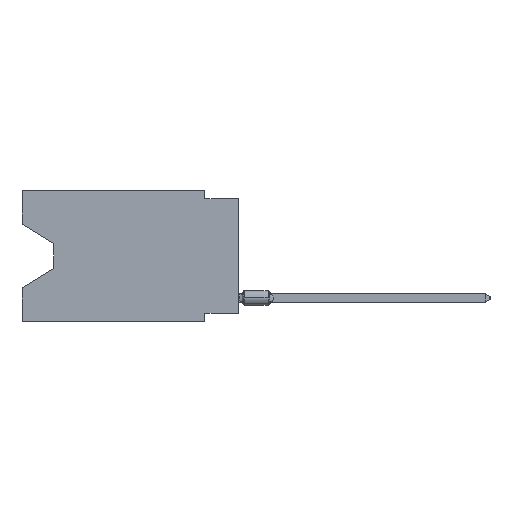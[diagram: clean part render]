
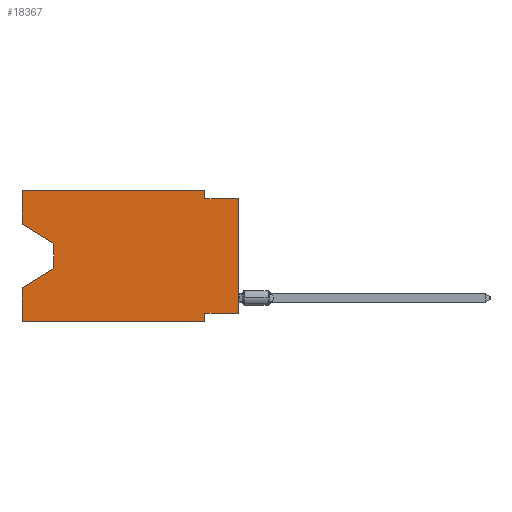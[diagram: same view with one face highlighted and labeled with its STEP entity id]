
A CAD part, left-side view. The second image highlights one B-rep face of the part: STEP entity #18367.
In plain terms, the highlighted planar face has unit normal (-1, 0, 0).
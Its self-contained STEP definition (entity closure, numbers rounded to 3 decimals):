
#168 = ORIENTED_EDGE ( 'NONE', *, *, #15667, .F. ) ;
#185 = VECTOR ( 'NONE', #19411, 1000. ) ;
#812 = VERTEX_POINT ( 'NONE', #38391 ) ;
#916 = VECTOR ( 'NONE', #42752, 1000. ) ;
#1492 = DIRECTION ( 'NONE',  ( 0., -1., 0. ) ) ;
#3178 = VERTEX_POINT ( 'NONE', #38609 ) ;
#3614 = CARTESIAN_POINT ( 'NONE',  ( 0., 0., -0.635 ) ) ;
#3881 = VERTEX_POINT ( 'NONE', #13965 ) ;
#4156 = EDGE_CURVE ( 'NONE', #30606, #30256, #38483, .T. ) ;
#4614 = CARTESIAN_POINT ( 'NONE',  ( 0., 16.383, -9.906 ) ) ;
#5006 = ORIENTED_EDGE ( 'NONE', *, *, #40846, .T. ) ;
#6402 = LINE ( 'NONE', #41507, #27598 ) ;
#7104 = VERTEX_POINT ( 'NONE', #14710 ) ;
#7480 = VECTOR ( 'NONE', #28845, 1000. ) ;
#7655 = LINE ( 'NONE', #31886, #916 ) ;
#8007 = EDGE_CURVE ( 'NONE', #7104, #30606, #35783, .T. ) ;
#8236 = CARTESIAN_POINT ( 'NONE',  ( 0., 16.383, -2.546 ) ) ;
#8937 = DIRECTION ( 'NONE',  ( 1., 0., 0. ) ) ;
#8999 = ORIENTED_EDGE ( 'NONE', *, *, #39989, .T. ) ;
#9164 = FACE_OUTER_BOUND ( 'NONE', #39672, .T. ) ;
#9329 = CARTESIAN_POINT ( 'NONE',  ( 0., 2.54, -9.271 ) ) ;
#9540 = ORIENTED_EDGE ( 'NONE', *, *, #4156, .F. ) ;
#9961 = ORIENTED_EDGE ( 'NONE', *, *, #20141, .F. ) ;
#10721 = DIRECTION ( 'NONE',  ( 0., -1., 0. ) ) ;
#10943 = LINE ( 'NONE', #42808, #21539 ) ;
#11065 = VECTOR ( 'NONE', #10721, 1000. ) ;
#12923 = VERTEX_POINT ( 'NONE', #24938 ) ;
#13878 = ORIENTED_EDGE ( 'NONE', *, *, #44050, .T. ) ;
#13965 = CARTESIAN_POINT ( 'NONE',  ( 0., 13.97, -4.013 ) ) ;
#14253 = DIRECTION ( 'NONE',  ( 0., -1., 0. ) ) ;
#14710 = CARTESIAN_POINT ( 'NONE',  ( 0., 2.54, 0. ) ) ;
#15667 = EDGE_CURVE ( 'NONE', #42163, #3178, #26783, .T. ) ;
#16546 = PLANE ( 'NONE',  #26722 ) ;
#16967 = ORIENTED_EDGE ( 'NONE', *, *, #26212, .T. ) ;
#17009 = CARTESIAN_POINT ( 'NONE',  ( 0., 16.383, 0. ) ) ;
#17024 = DIRECTION ( 'NONE',  ( 0., 0.855, -0.519 ) ) ;
#17394 = VECTOR ( 'NONE', #34828, 1000. ) ;
#17498 = LINE ( 'NONE', #27440, #17394 ) ;
#18367 = ADVANCED_FACE ( 'NONE', ( #9164 ), #16546, .F. ) ;
#19096 = ORIENTED_EDGE ( 'NONE', *, *, #8007, .F. ) ;
#19411 = DIRECTION ( 'NONE',  ( 0., 0., 1. ) ) ;
#19811 = EDGE_CURVE ( 'NONE', #23312, #12923, #17498, .T. ) ;
#20141 = EDGE_CURVE ( 'NONE', #812, #43553, #26247, .T. ) ;
#21539 = VECTOR ( 'NONE', #39777, 1000. ) ;
#21571 = LINE ( 'NONE', #42586, #11065 ) ;
#22924 = ORIENTED_EDGE ( 'NONE', *, *, #26256, .F. ) ;
#23024 = DIRECTION ( 'NONE',  ( 0., 0., 1. ) ) ;
#23312 = VERTEX_POINT ( 'NONE', #9329 ) ;
#24254 = VECTOR ( 'NONE', #14253, 1000. ) ;
#24682 = CARTESIAN_POINT ( 'NONE',  ( 0., 2.54, -0.635 ) ) ;
#24904 = CARTESIAN_POINT ( 'NONE',  ( 0., 16.383, 0. ) ) ;
#24938 = CARTESIAN_POINT ( 'NONE',  ( 0., 2.54, -9.906 ) ) ;
#26212 = EDGE_CURVE ( 'NONE', #32530, #3178, #30872, .T. ) ;
#26247 = LINE ( 'NONE', #33397, #43256 ) ;
#26256 = EDGE_CURVE ( 'NONE', #35920, #23312, #6402, .T. ) ;
#26574 = VECTOR ( 'NONE', #43104, 1000. ) ;
#26722 = AXIS2_PLACEMENT_3D ( 'NONE', #17009, #8937, #27160 ) ;
#26783 = LINE ( 'NONE', #40863, #185 ) ;
#27160 = DIRECTION ( 'NONE',  ( 0., 0., -1. ) ) ;
#27440 = CARTESIAN_POINT ( 'NONE',  ( 0., 2.54, -9.906 ) ) ;
#27598 = VECTOR ( 'NONE', #35246, 1000. ) ;
#28845 = DIRECTION ( 'NONE',  ( 0., 0., -1. ) ) ;
#28856 = VECTOR ( 'NONE', #1492, 1000. ) ;
#29005 = LINE ( 'NONE', #8236, #26574 ) ;
#29412 = CARTESIAN_POINT ( 'NONE',  ( 0., 16.383, 0. ) ) ;
#29973 = CARTESIAN_POINT ( 'NONE',  ( 0., 13.97, -5.893 ) ) ;
#30256 = VERTEX_POINT ( 'NONE', #39338 ) ;
#30606 = VERTEX_POINT ( 'NONE', #24682 ) ;
#30872 = LINE ( 'NONE', #45644, #37961 ) ;
#31886 = CARTESIAN_POINT ( 'NONE',  ( 0., 13.97, -4.013 ) ) ;
#32530 = VERTEX_POINT ( 'NONE', #29973 ) ;
#33397 = CARTESIAN_POINT ( 'NONE',  ( 0., 16.383, 0. ) ) ;
#34828 = DIRECTION ( 'NONE',  ( 0., 0., -1. ) ) ;
#35246 = DIRECTION ( 'NONE',  ( 0., 1., 0. ) ) ;
#35255 = EDGE_CURVE ( 'NONE', #43553, #7104, #44430, .T. ) ;
#35783 = LINE ( 'NONE', #39694, #7480 ) ;
#35920 = VERTEX_POINT ( 'NONE', #39282 ) ;
#35976 = EDGE_CURVE ( 'NONE', #3881, #32530, #7655, .T. ) ;
#37693 = ORIENTED_EDGE ( 'NONE', *, *, #19811, .F. ) ;
#37961 = VECTOR ( 'NONE', #17024, 1000. ) ;
#38391 = CARTESIAN_POINT ( 'NONE',  ( 0., 16.383, -2.546 ) ) ;
#38483 = LINE ( 'NONE', #3614, #24254 ) ;
#38609 = CARTESIAN_POINT ( 'NONE',  ( 0., 16.383, -7.36 ) ) ;
#39282 = CARTESIAN_POINT ( 'NONE',  ( 0., 0., -9.271 ) ) ;
#39338 = CARTESIAN_POINT ( 'NONE',  ( 0., 0., -0.635 ) ) ;
#39672 = EDGE_LOOP ( 'NONE', ( #5006, #41827, #16967, #168, #8999, #37693, #22924, #13878, #9540, #19096, #45221, #9961 ) ) ;
#39694 = CARTESIAN_POINT ( 'NONE',  ( 0., 2.54, 0. ) ) ;
#39777 = DIRECTION ( 'NONE',  ( 0., 0., 1. ) ) ;
#39989 = EDGE_CURVE ( 'NONE', #42163, #12923, #21571, .T. ) ;
#40846 = EDGE_CURVE ( 'NONE', #812, #3881, #29005, .T. ) ;
#40863 = CARTESIAN_POINT ( 'NONE',  ( 0., 16.383, 0. ) ) ;
#41507 = CARTESIAN_POINT ( 'NONE',  ( 0., 0., -9.271 ) ) ;
#41827 = ORIENTED_EDGE ( 'NONE', *, *, #35976, .T. ) ;
#42163 = VERTEX_POINT ( 'NONE', #4614 ) ;
#42586 = CARTESIAN_POINT ( 'NONE',  ( 0., 16.383, -9.906 ) ) ;
#42752 = DIRECTION ( 'NONE',  ( 0., 0., -1. ) ) ;
#42808 = CARTESIAN_POINT ( 'NONE',  ( 0., 0., 0. ) ) ;
#43104 = DIRECTION ( 'NONE',  ( 0., -0.855, -0.519 ) ) ;
#43256 = VECTOR ( 'NONE', #23024, 1000. ) ;
#43553 = VERTEX_POINT ( 'NONE', #24904 ) ;
#44050 = EDGE_CURVE ( 'NONE', #35920, #30256, #10943, .T. ) ;
#44430 = LINE ( 'NONE', #29412, #28856 ) ;
#45221 = ORIENTED_EDGE ( 'NONE', *, *, #35255, .F. ) ;
#45644 = CARTESIAN_POINT ( 'NONE',  ( 0., 13.97, -5.893 ) ) ;
